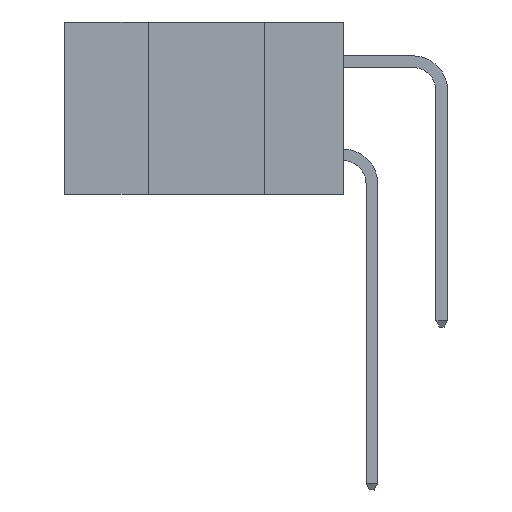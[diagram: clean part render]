
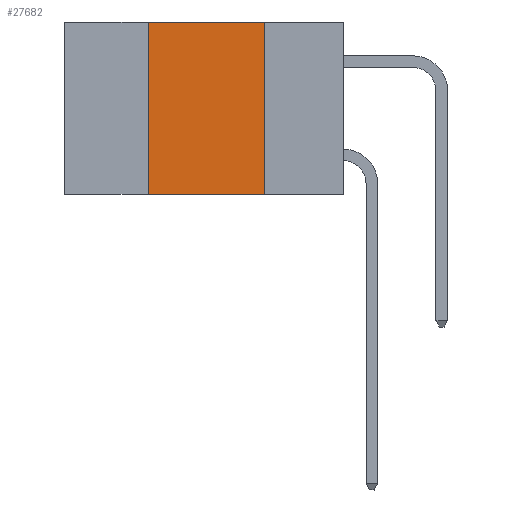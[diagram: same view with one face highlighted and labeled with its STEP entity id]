
A CAD part, left-side view. The second image highlights one B-rep face of the part: STEP entity #27682.
In plain terms, the highlighted planar face has unit normal (-1, 0, 0).
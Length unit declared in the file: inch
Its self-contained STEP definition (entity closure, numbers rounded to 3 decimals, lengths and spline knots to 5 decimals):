
#671 = DIRECTION ( 'NONE',  ( 1., 0., 0. ) ) ;
#896 = LINE ( 'NONE', #15372, #8860 ) ;
#1792 = VERTEX_POINT ( 'NONE', #32130 ) ;
#2042 = DIRECTION ( 'NONE',  ( 0., -1., 0. ) ) ;
#4250 = ORIENTED_EDGE ( 'NONE', *, *, #11822, .F. ) ;
#6776 = VECTOR ( 'NONE', #21870, 39.37008 ) ;
#8059 = VECTOR ( 'NONE', #18924, 39.37008 ) ;
#8288 = CARTESIAN_POINT ( 'NONE',  ( 0., 0.17, 0. ) ) ;
#8860 = VECTOR ( 'NONE', #2042, 39.37008 ) ;
#10042 = ORIENTED_EDGE ( 'NONE', *, *, #32858, .F. ) ;
#10060 = DIRECTION ( 'NONE',  ( 0., 0., 1. ) ) ;
#10255 = VERTEX_POINT ( 'NONE', #29790 ) ;
#11343 = PLANE ( 'NONE',  #20708 ) ;
#11822 = EDGE_CURVE ( 'NONE', #13662, #10255, #23500, .T. ) ;
#12487 = EDGE_CURVE ( 'NONE', #13662, #1792, #896, .T. ) ;
#13416 = CARTESIAN_POINT ( 'NONE',  ( 0., 0.17, 0. ) ) ;
#13662 = VERTEX_POINT ( 'NONE', #18270 ) ;
#15169 = LINE ( 'NONE', #8288, #8059 ) ;
#15372 = CARTESIAN_POINT ( 'NONE',  ( 0., 0.6, -0.37 ) ) ;
#18270 = CARTESIAN_POINT ( 'NONE',  ( 0., 0.42, -0.37 ) ) ;
#18924 = DIRECTION ( 'NONE',  ( 0., 0., -1. ) ) ;
#19181 = CARTESIAN_POINT ( 'NONE',  ( 0., 0.6, 0. ) ) ;
#19367 = DIRECTION ( 'NONE',  ( 0., 0., -1. ) ) ;
#20708 = AXIS2_PLACEMENT_3D ( 'NONE', #21935, #671, #19367 ) ;
#21826 = LINE ( 'NONE', #19181, #6776 ) ;
#21870 = DIRECTION ( 'NONE',  ( 0., -1., 0. ) ) ;
#21935 = CARTESIAN_POINT ( 'NONE',  ( 0., 0.6, 0. ) ) ;
#22527 = EDGE_CURVE ( 'NONE', #28589, #1792, #15169, .T. ) ;
#23500 = LINE ( 'NONE', #33892, #29610 ) ;
#25548 = EDGE_LOOP ( 'NONE', ( #29016, #10042, #4250, #32546 ) ) ;
#27682 = ADVANCED_FACE ( 'NONE', ( #32660 ), #11343, .F. ) ;
#28589 = VERTEX_POINT ( 'NONE', #13416 ) ;
#29016 = ORIENTED_EDGE ( 'NONE', *, *, #22527, .F. ) ;
#29610 = VECTOR ( 'NONE', #10060, 39.37008 ) ;
#29790 = CARTESIAN_POINT ( 'NONE',  ( 0., 0.42, 0. ) ) ;
#32130 = CARTESIAN_POINT ( 'NONE',  ( 0., 0.17, -0.37 ) ) ;
#32546 = ORIENTED_EDGE ( 'NONE', *, *, #12487, .T. ) ;
#32660 = FACE_OUTER_BOUND ( 'NONE', #25548, .T. ) ;
#32858 = EDGE_CURVE ( 'NONE', #10255, #28589, #21826, .T. ) ;
#33892 = CARTESIAN_POINT ( 'NONE',  ( 0., 0.42, 0. ) ) ;
